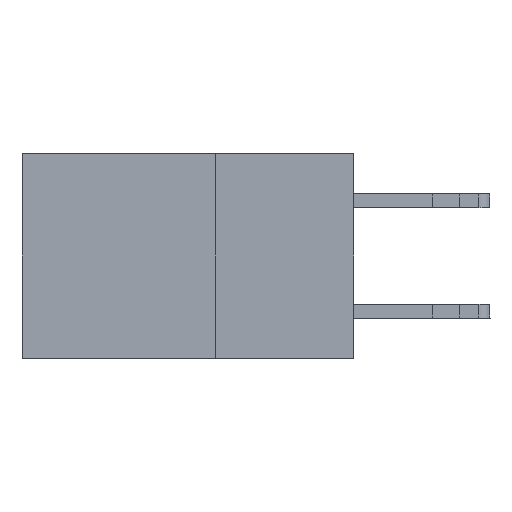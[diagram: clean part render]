
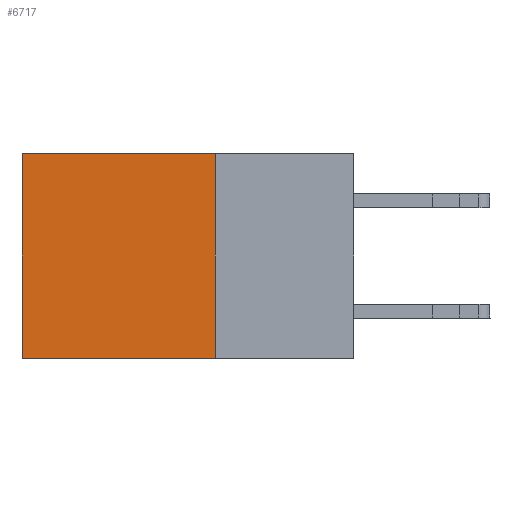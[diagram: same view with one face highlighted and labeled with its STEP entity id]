
A CAD part, left-side view. The second image highlights one B-rep face of the part: STEP entity #6717.
In plain terms, the highlighted planar face has unit normal (-1, 0, 0).
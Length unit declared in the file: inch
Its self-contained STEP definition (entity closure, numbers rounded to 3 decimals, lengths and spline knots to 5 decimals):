
#891 = VECTOR ( 'NONE', #30284, 39.37008 ) ;
#2371 = LINE ( 'NONE', #10149, #8489 ) ;
#5034 = VERTEX_POINT ( 'NONE', #30350 ) ;
#5091 = FACE_OUTER_BOUND ( 'NONE', #21556, .T. ) ;
#5710 = ORIENTED_EDGE ( 'NONE', *, *, #8371, .T. ) ;
#5858 = EDGE_CURVE ( 'NONE', #5034, #14465, #18808, .T. ) ;
#6717 = ADVANCED_FACE ( 'NONE', ( #5091 ), #12060, .F. ) ;
#7812 = ORIENTED_EDGE ( 'NONE', *, *, #11502, .T. ) ;
#8371 = EDGE_CURVE ( 'NONE', #5034, #25988, #19628, .T. ) ;
#8489 = VECTOR ( 'NONE', #17494, 39.37008 ) ;
#9136 = ORIENTED_EDGE ( 'NONE', *, *, #5858, .F. ) ;
#9311 = DIRECTION ( 'NONE',  ( 1., 0., 0. ) ) ;
#10149 = CARTESIAN_POINT ( 'NONE',  ( 0.2875, 0.25, -0.37 ) ) ;
#11502 = EDGE_CURVE ( 'NONE', #25988, #24922, #23325, .T. ) ;
#12060 = PLANE ( 'NONE',  #16752 ) ;
#13030 = CARTESIAN_POINT ( 'NONE',  ( 0.2875, 0.25, 0. ) ) ;
#14293 = ORIENTED_EDGE ( 'NONE', *, *, #31593, .F. ) ;
#14465 = VERTEX_POINT ( 'NONE', #14520 ) ;
#14520 = CARTESIAN_POINT ( 'NONE',  ( 0.2875, 0.25, -0.37 ) ) ;
#16354 = DIRECTION ( 'NONE',  ( 0., 1., 0. ) ) ;
#16557 = DIRECTION ( 'NONE',  ( 0., 0., -1. ) ) ;
#16752 = AXIS2_PLACEMENT_3D ( 'NONE', #18944, #9311, #19049 ) ;
#17196 = CARTESIAN_POINT ( 'NONE',  ( 0.2875, 0.6, 0. ) ) ;
#17494 = DIRECTION ( 'NONE',  ( 0., 1., 0. ) ) ;
#18410 = CARTESIAN_POINT ( 'NONE',  ( 0.2875, 0.6, 0. ) ) ;
#18808 = LINE ( 'NONE', #13030, #891 ) ;
#18944 = CARTESIAN_POINT ( 'NONE',  ( 0.2875, 0.25, 0. ) ) ;
#19049 = DIRECTION ( 'NONE',  ( 0., 0., -1. ) ) ;
#19628 = LINE ( 'NONE', #23780, #20749 ) ;
#20749 = VECTOR ( 'NONE', #16354, 39.37008 ) ;
#21556 = EDGE_LOOP ( 'NONE', ( #7812, #14293, #9136, #5710 ) ) ;
#23325 = LINE ( 'NONE', #18410, #29037 ) ;
#23780 = CARTESIAN_POINT ( 'NONE',  ( 0.2875, 0.25, 0. ) ) ;
#24922 = VERTEX_POINT ( 'NONE', #28880 ) ;
#25988 = VERTEX_POINT ( 'NONE', #17196 ) ;
#28880 = CARTESIAN_POINT ( 'NONE',  ( 0.2875, 0.6, -0.37 ) ) ;
#29037 = VECTOR ( 'NONE', #16557, 39.37008 ) ;
#30284 = DIRECTION ( 'NONE',  ( 0., 0., -1. ) ) ;
#30350 = CARTESIAN_POINT ( 'NONE',  ( 0.2875, 0.25, 0. ) ) ;
#31593 = EDGE_CURVE ( 'NONE', #14465, #24922, #2371, .T. ) ;
